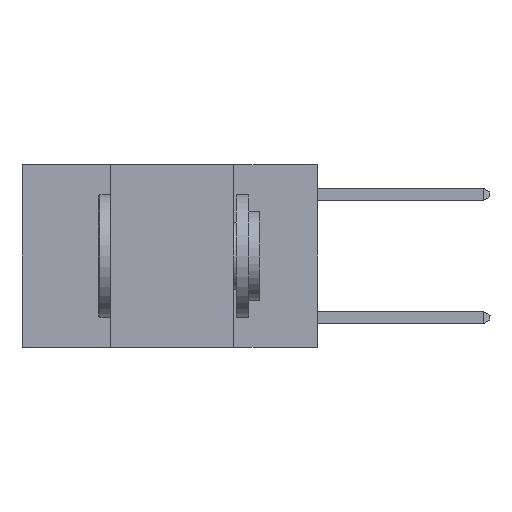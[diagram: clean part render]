
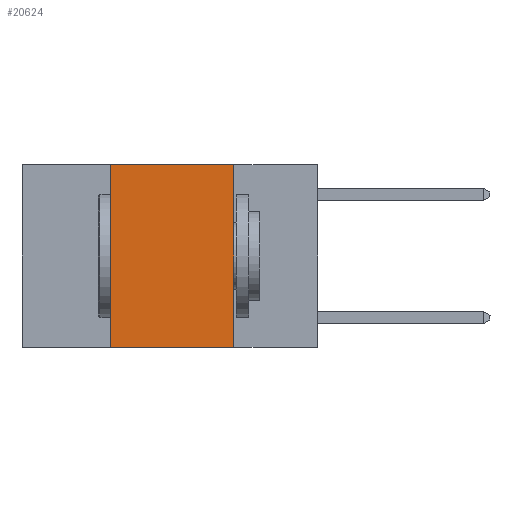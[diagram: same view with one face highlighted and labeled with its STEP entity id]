
A CAD part, left-side view. The second image highlights one B-rep face of the part: STEP entity #20624.
In plain terms, the highlighted planar face has unit normal (-1, 0, 0).
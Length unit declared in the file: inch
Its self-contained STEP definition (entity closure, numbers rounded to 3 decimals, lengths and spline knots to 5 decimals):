
#423 = PLANE ( 'NONE',  #5561 ) ;
#725 = VECTOR ( 'NONE', #16530, 39.37008 ) ;
#2620 = VECTOR ( 'NONE', #18232, 39.37008 ) ;
#2714 = CARTESIAN_POINT ( 'NONE',  ( 0., 0.6, 0. ) ) ;
#3006 = EDGE_CURVE ( 'NONE', #11334, #24768, #24902, .T. ) ;
#3425 = ORIENTED_EDGE ( 'NONE', *, *, #21513, .F. ) ;
#4277 = VECTOR ( 'NONE', #6053, 39.37008 ) ;
#4992 = DIRECTION ( 'NONE',  ( 0., 0., -1. ) ) ;
#5101 = EDGE_CURVE ( 'NONE', #10154, #24768, #17939, .T. ) ;
#5561 = AXIS2_PLACEMENT_3D ( 'NONE', #2714, #18350, #4992 ) ;
#6053 = DIRECTION ( 'NONE',  ( 0., 0., 1. ) ) ;
#6656 = CARTESIAN_POINT ( 'NONE',  ( 0., 0.42, -0.37 ) ) ;
#8307 = ORIENTED_EDGE ( 'NONE', *, *, #3006, .T. ) ;
#10154 = VERTEX_POINT ( 'NONE', #15609 ) ;
#11334 = VERTEX_POINT ( 'NONE', #6656 ) ;
#11906 = ORIENTED_EDGE ( 'NONE', *, *, #22385, .F. ) ;
#13246 = CARTESIAN_POINT ( 'NONE',  ( 0., 0.6, 0. ) ) ;
#14627 = ORIENTED_EDGE ( 'NONE', *, *, #5101, .F. ) ;
#14690 = EDGE_LOOP ( 'NONE', ( #14627, #11906, #3425, #8307 ) ) ;
#15469 = DIRECTION ( 'NONE',  ( 0., -1., 0. ) ) ;
#15609 = CARTESIAN_POINT ( 'NONE',  ( 0., 0.17, 0. ) ) ;
#15996 = CARTESIAN_POINT ( 'NONE',  ( 0., 0.6, -0.37 ) ) ;
#16530 = DIRECTION ( 'NONE',  ( 0., 0., -1. ) ) ;
#17939 = LINE ( 'NONE', #20864, #725 ) ;
#18221 = LINE ( 'NONE', #13246, #24115 ) ;
#18232 = DIRECTION ( 'NONE',  ( 0., -1., 0. ) ) ;
#18350 = DIRECTION ( 'NONE',  ( 1., 0., 0. ) ) ;
#20624 = ADVANCED_FACE ( 'NONE', ( #27205 ), #423, .F. ) ;
#20864 = CARTESIAN_POINT ( 'NONE',  ( 0., 0.17, 0. ) ) ;
#21383 = VERTEX_POINT ( 'NONE', #25653 ) ;
#21513 = EDGE_CURVE ( 'NONE', #11334, #21383, #27847, .T. ) ;
#22385 = EDGE_CURVE ( 'NONE', #21383, #10154, #18221, .T. ) ;
#24115 = VECTOR ( 'NONE', #15469, 39.37008 ) ;
#24768 = VERTEX_POINT ( 'NONE', #28022 ) ;
#24902 = LINE ( 'NONE', #15996, #2620 ) ;
#25653 = CARTESIAN_POINT ( 'NONE',  ( 0., 0.42, 0. ) ) ;
#26022 = CARTESIAN_POINT ( 'NONE',  ( 0., 0.42, 0. ) ) ;
#27205 = FACE_OUTER_BOUND ( 'NONE', #14690, .T. ) ;
#27847 = LINE ( 'NONE', #26022, #4277 ) ;
#28022 = CARTESIAN_POINT ( 'NONE',  ( 0., 0.17, -0.37 ) ) ;
